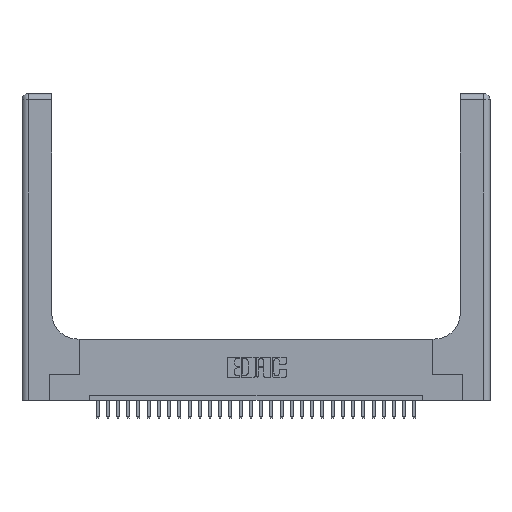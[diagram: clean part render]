
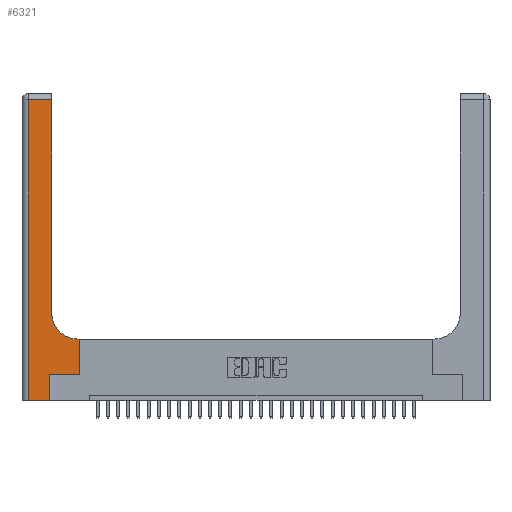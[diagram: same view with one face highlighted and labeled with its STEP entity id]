
A CAD part, top view. The second image highlights one B-rep face of the part: STEP entity #6321.
In plain terms, the highlighted planar face has unit normal (0, 0, 1).
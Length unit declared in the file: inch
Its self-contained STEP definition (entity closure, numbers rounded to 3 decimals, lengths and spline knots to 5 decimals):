
#27 = VERTEX_POINT ( 'NONE', #5129 ) ;
#1001 = VERTEX_POINT ( 'NONE', #18834 ) ;
#1044 = VERTEX_POINT ( 'NONE', #13863 ) ;
#2008 = EDGE_CURVE ( 'NONE', #11732, #1044, #30054, .T. ) ;
#2699 = CARTESIAN_POINT ( 'NONE',  ( 0., 0., 0.37 ) ) ;
#2708 = VECTOR ( 'NONE', #28473, 39.37008 ) ;
#3943 = EDGE_CURVE ( 'NONE', #23251, #14331, #6156, .T. ) ;
#4264 = DIRECTION ( 'NONE',  ( -1., 0., 0. ) ) ;
#4373 = CARTESIAN_POINT ( 'NONE',  ( 0.5585, 0.25, 0.37 ) ) ;
#4719 = DIRECTION ( 'NONE',  ( -1., 0., 0. ) ) ;
#4733 = CARTESIAN_POINT ( 'NONE',  ( 0.269, 0., 0.37 ) ) ;
#4937 = LINE ( 'NONE', #2699, #9411 ) ;
#5129 = CARTESIAN_POINT ( 'NONE',  ( 0.5585, 0.6, 0.37 ) ) ;
#5229 = ORIENTED_EDGE ( 'NONE', *, *, #16912, .T. ) ;
#5758 = EDGE_CURVE ( 'NONE', #28280, #20881, #20525, .T. ) ;
#6028 = ORIENTED_EDGE ( 'NONE', *, *, #2008, .T. ) ;
#6128 = DIRECTION ( 'NONE',  ( -1., 0., 0. ) ) ;
#6156 = LINE ( 'NONE', #18360, #10625 ) ;
#6306 = ORIENTED_EDGE ( 'NONE', *, *, #10872, .T. ) ;
#6321 = ADVANCED_FACE ( 'NONE', ( #10119 ), #19718, .F. ) ;
#6587 = EDGE_CURVE ( 'NONE', #14331, #28280, #4937, .T. ) ;
#6955 = EDGE_CURVE ( 'NONE', #1001, #27, #23445, .T. ) ;
#7912 = CARTESIAN_POINT ( 'NONE',  ( 0., 3., 0.37 ) ) ;
#8012 = EDGE_LOOP ( 'NONE', ( #8722, #6306, #10533, #15827, #15389, #5229, #21493, #8353, #6028 ) ) ;
#8019 = EDGE_CURVE ( 'NONE', #1044, #25078, #12657, .T. ) ;
#8066 = AXIS2_PLACEMENT_3D ( 'NONE', #7912, #12675, #6128 ) ;
#8353 = ORIENTED_EDGE ( 'NONE', *, *, #30589, .T. ) ;
#8722 = ORIENTED_EDGE ( 'NONE', *, *, #8019, .T. ) ;
#8869 = LINE ( 'NONE', #29225, #23679 ) ;
#9124 = CARTESIAN_POINT ( 'NONE',  ( 0.5415, 0.85, 0.37 ) ) ;
#9411 = VECTOR ( 'NONE', #26416, 39.37008 ) ;
#9433 = DIRECTION ( 'NONE',  ( 1., 0., 0. ) ) ;
#9671 = CARTESIAN_POINT ( 'NONE',  ( 0.2915, 2.94, 0.37 ) ) ;
#9765 = CARTESIAN_POINT ( 'NONE',  ( 0.269, 0.25, 0.37 ) ) ;
#10119 = FACE_OUTER_BOUND ( 'NONE', #8012, .T. ) ;
#10533 = ORIENTED_EDGE ( 'NONE', *, *, #3943, .T. ) ;
#10625 = VECTOR ( 'NONE', #11323, 39.37008 ) ;
#10872 = EDGE_CURVE ( 'NONE', #25078, #23251, #26172, .T. ) ;
#10942 = LINE ( 'NONE', #26359, #30602 ) ;
#11240 = CARTESIAN_POINT ( 'NONE',  ( 0., 2.94, 0.37 ) ) ;
#11323 = DIRECTION ( 'NONE',  ( 0., -1., 0. ) ) ;
#11732 = VERTEX_POINT ( 'NONE', #16934 ) ;
#12544 = DIRECTION ( 'NONE',  ( 1., 0., 0. ) ) ;
#12657 = LINE ( 'NONE', #20829, #28591 ) ;
#12675 = DIRECTION ( 'NONE',  ( 0., 0., -1. ) ) ;
#13863 = CARTESIAN_POINT ( 'NONE',  ( 0.2915, 0.85, 0.37 ) ) ;
#14257 = DIRECTION ( 'NONE',  ( 0., 1., 0. ) ) ;
#14331 = VERTEX_POINT ( 'NONE', #23921 ) ;
#15389 = ORIENTED_EDGE ( 'NONE', *, *, #5758, .T. ) ;
#15827 = ORIENTED_EDGE ( 'NONE', *, *, #6587, .T. ) ;
#16912 = EDGE_CURVE ( 'NONE', #20881, #1001, #8869, .T. ) ;
#16934 = CARTESIAN_POINT ( 'NONE',  ( 0.5415, 0.6, 0.37 ) ) ;
#18360 = CARTESIAN_POINT ( 'NONE',  ( 0.06, 3., 0.37 ) ) ;
#18834 = CARTESIAN_POINT ( 'NONE',  ( 0.5585, 0.25, 0.37 ) ) ;
#18898 = DIRECTION ( 'NONE',  ( 0., 1., 0. ) ) ;
#19718 = PLANE ( 'NONE',  #8066 ) ;
#20457 = CARTESIAN_POINT ( 'NONE',  ( 0.269, 0., 0.37 ) ) ;
#20500 = AXIS2_PLACEMENT_3D ( 'NONE', #9124, #21322, #9433 ) ;
#20525 = LINE ( 'NONE', #4733, #2708 ) ;
#20829 = CARTESIAN_POINT ( 'NONE',  ( 0.2915, 3., 0.37 ) ) ;
#20881 = VERTEX_POINT ( 'NONE', #9765 ) ;
#21322 = DIRECTION ( 'NONE',  ( 0., 0., -1. ) ) ;
#21493 = ORIENTED_EDGE ( 'NONE', *, *, #6955, .T. ) ;
#23251 = VERTEX_POINT ( 'NONE', #25389 ) ;
#23445 = LINE ( 'NONE', #4373, #29396 ) ;
#23679 = VECTOR ( 'NONE', #12544, 39.37008 ) ;
#23921 = CARTESIAN_POINT ( 'NONE',  ( 0.06, 0., 0.37 ) ) ;
#24315 = VECTOR ( 'NONE', #4264, 39.37008 ) ;
#25078 = VERTEX_POINT ( 'NONE', #9671 ) ;
#25389 = CARTESIAN_POINT ( 'NONE',  ( 0.06, 2.94, 0.37 ) ) ;
#26172 = LINE ( 'NONE', #11240, #24315 ) ;
#26359 = CARTESIAN_POINT ( 'NONE',  ( 0.2915, 0.6, 0.37 ) ) ;
#26416 = DIRECTION ( 'NONE',  ( 1., 0., 0. ) ) ;
#28280 = VERTEX_POINT ( 'NONE', #20457 ) ;
#28473 = DIRECTION ( 'NONE',  ( 0., 1., 0. ) ) ;
#28591 = VECTOR ( 'NONE', #14257, 39.37008 ) ;
#29225 = CARTESIAN_POINT ( 'NONE',  ( 0.269, 0.25, 0.37 ) ) ;
#29396 = VECTOR ( 'NONE', #18898, 39.37008 ) ;
#30054 = CIRCLE ( 'NONE', #20500, 0.25 ) ;
#30589 = EDGE_CURVE ( 'NONE', #27, #11732, #10942, .T. ) ;
#30602 = VECTOR ( 'NONE', #4719, 39.37008 ) ;
